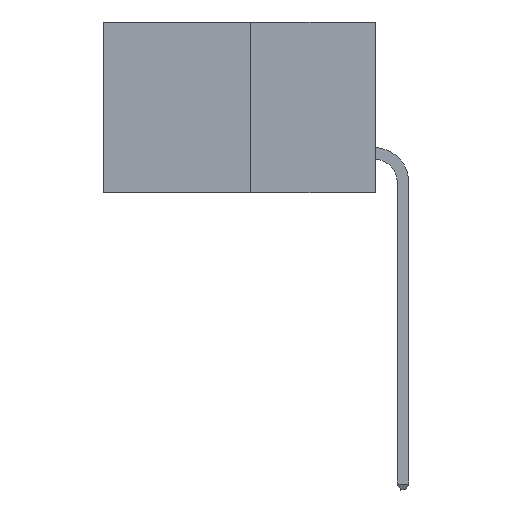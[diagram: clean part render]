
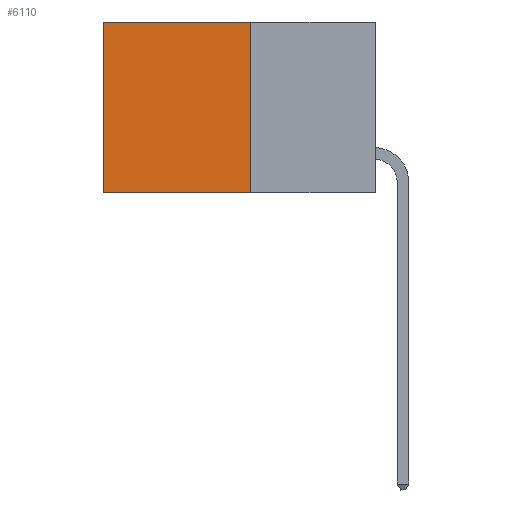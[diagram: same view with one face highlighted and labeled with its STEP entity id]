
A CAD part, left-side view. The second image highlights one B-rep face of the part: STEP entity #6110.
In plain terms, the highlighted planar face has unit normal (-1, 0, 0).
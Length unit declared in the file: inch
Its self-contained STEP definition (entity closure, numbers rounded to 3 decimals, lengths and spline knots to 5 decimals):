
#396 = VERTEX_POINT ( 'NONE', #6858 ) ;
#1952 = CARTESIAN_POINT ( 'NONE',  ( 0.277, 0.27, -0.37 ) ) ;
#2038 = VERTEX_POINT ( 'NONE', #23594 ) ;
#2506 = CARTESIAN_POINT ( 'NONE',  ( 0.277, 0.27, -0.37 ) ) ;
#2815 = LINE ( 'NONE', #25683, #14589 ) ;
#3262 = PLANE ( 'NONE',  #9588 ) ;
#3366 = DIRECTION ( 'NONE',  ( 1., 0., 0. ) ) ;
#3392 = VERTEX_POINT ( 'NONE', #19575 ) ;
#5142 = CARTESIAN_POINT ( 'NONE',  ( 0.277, 0.27, -0.37 ) ) ;
#6110 = ADVANCED_FACE ( 'NONE', ( #21358 ), #3262, .F. ) ;
#6858 = CARTESIAN_POINT ( 'NONE',  ( 0.277, 0.59, 0. ) ) ;
#7274 = ORIENTED_EDGE ( 'NONE', *, *, #19436, .T. ) ;
#7478 = ORIENTED_EDGE ( 'NONE', *, *, #20723, .F. ) ;
#7911 = LINE ( 'NONE', #2506, #13434 ) ;
#8336 = VERTEX_POINT ( 'NONE', #1952 ) ;
#9588 = AXIS2_PLACEMENT_3D ( 'NONE', #26834, #3366, #19775 ) ;
#10274 = EDGE_CURVE ( 'NONE', #8336, #2038, #29164, .T. ) ;
#12814 = LINE ( 'NONE', #14611, #16868 ) ;
#13434 = VECTOR ( 'NONE', #21247, 39.37008 ) ;
#14589 = VECTOR ( 'NONE', #23296, 39.37008 ) ;
#14611 = CARTESIAN_POINT ( 'NONE',  ( 0.277, 0.59, -0.37 ) ) ;
#15375 = EDGE_LOOP ( 'NONE', ( #25897, #23316, #7478, #7274 ) ) ;
#16670 = VECTOR ( 'NONE', #23949, 39.37008 ) ;
#16868 = VECTOR ( 'NONE', #23916, 39.37008 ) ;
#18117 = EDGE_CURVE ( 'NONE', #396, #2038, #12814, .T. ) ;
#19436 = EDGE_CURVE ( 'NONE', #3392, #396, #2815, .T. ) ;
#19575 = CARTESIAN_POINT ( 'NONE',  ( 0.277, 0.27, 0. ) ) ;
#19775 = DIRECTION ( 'NONE',  ( 0., 0., -1. ) ) ;
#20723 = EDGE_CURVE ( 'NONE', #3392, #8336, #7911, .T. ) ;
#21247 = DIRECTION ( 'NONE',  ( 0., 0., -1. ) ) ;
#21358 = FACE_OUTER_BOUND ( 'NONE', #15375, .T. ) ;
#23296 = DIRECTION ( 'NONE',  ( 0., 1., 0. ) ) ;
#23316 = ORIENTED_EDGE ( 'NONE', *, *, #10274, .F. ) ;
#23594 = CARTESIAN_POINT ( 'NONE',  ( 0.277, 0.59, -0.37 ) ) ;
#23916 = DIRECTION ( 'NONE',  ( 0., 0., -1. ) ) ;
#23949 = DIRECTION ( 'NONE',  ( 0., 1., 0. ) ) ;
#25683 = CARTESIAN_POINT ( 'NONE',  ( 0.277, 0.27, 0. ) ) ;
#25897 = ORIENTED_EDGE ( 'NONE', *, *, #18117, .T. ) ;
#26834 = CARTESIAN_POINT ( 'NONE',  ( 0.277, 0.27, -0.37 ) ) ;
#29164 = LINE ( 'NONE', #5142, #16670 ) ;
